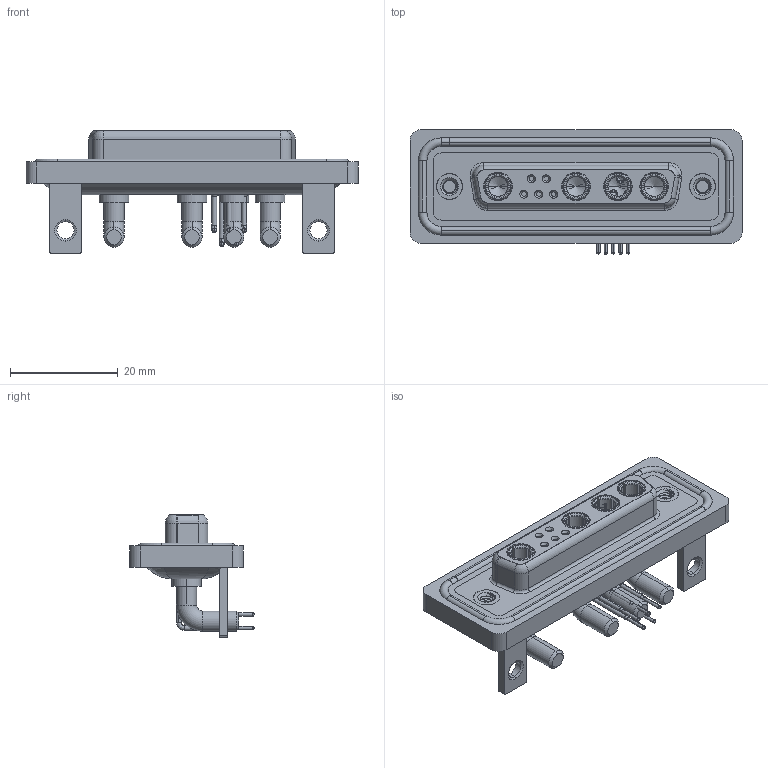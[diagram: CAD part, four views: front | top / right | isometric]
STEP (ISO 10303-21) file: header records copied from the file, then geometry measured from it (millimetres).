
FILE_DESCRIPTION (( 'STEP AP203' ), '1' );
FILE_NAME ('630W9W4-340-4N4.STEP', '2024-04-12T01:11:12', ( '' ), ( '' ), 'SwSTEP 2.0', 'SolidWorks 2023', '' );
FILE_SCHEMA (( 'CONFIG_CONTROL_DESIGN' ));
Length unit declared in the file: millimetre
Products named in the file (10): 630Combo Threaded Rivet_2; 630Combo Shell Rear_25 Contacts; 630Combo Waterproof Housing_25 Contacts; 630Combo Shell Front_25 Contacts; 630Combo Contact Row 2_50 Contacts; Power Socket_40A RA; 630Combo Contact Row 1_50 Contacts; 630W9W4-340-4N4; 630Combo Stabilizer Bracket_50 Contacts; 630Combo Housing_9W4
Assembly tree (17 placements, depth 2):
  630W9W4-340-4N4
    630Combo Housing_9W4
    630Combo Shell Front_25 Contacts
    630Combo Shell Rear_25 Contacts
    630Combo Threaded Rivet_2  x2
    630Combo Stabilizer Bracket_50 Contacts  x2
    Power Socket_40A RA  x4
    630Combo Contact Row 1_50 Contacts  x2
    630Combo Contact Row 2_50 Contacts  x3
    630Combo Waterproof Housing_25 Contacts
Bounding box: 61.75 x 23.12 x 22.8 mm (x, y, z)
Volume: 9108.9 mm3; surface area: 14957.3 mm2
Topology: 22 solids, 22 shells, 1011 faces, 2592 edges, 1647 vertices
Faces by surface type: cylinder 427, plane 316, cone 139, torus 95, bspline 34
Entity records: 21841 total; most frequent: CARTESIAN_POINT 5530, DIRECTION 3352, ORIENTED_EDGE 3056, EDGE_CURVE 1528, AXIS2_PLACEMENT_3D 1354, VERTEX_POINT 977, CIRCLE 735, EDGE_LOOP 695
